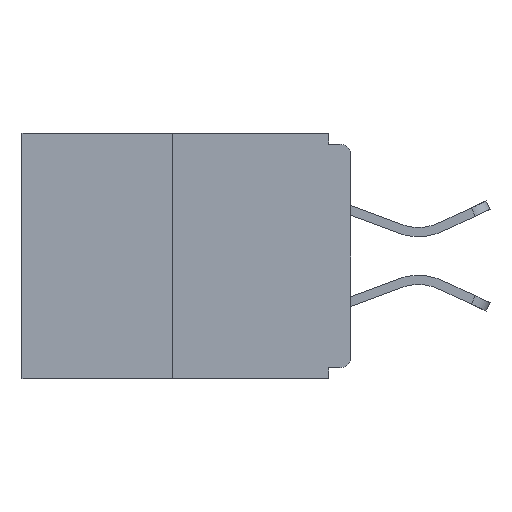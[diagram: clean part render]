
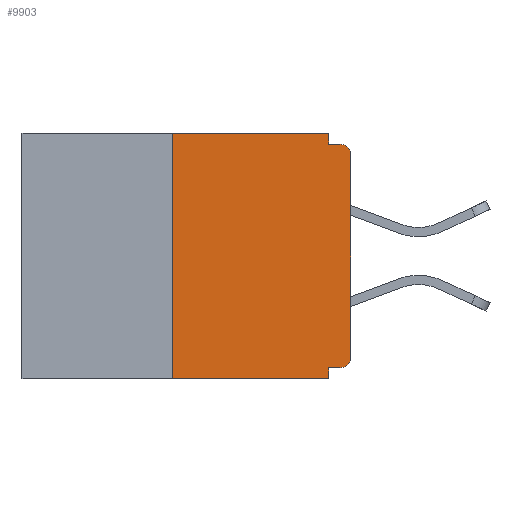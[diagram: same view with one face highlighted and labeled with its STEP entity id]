
A CAD part, left-side view. The second image highlights one B-rep face of the part: STEP entity #9903.
In plain terms, the highlighted planar face has unit normal (-1, 0, 0).
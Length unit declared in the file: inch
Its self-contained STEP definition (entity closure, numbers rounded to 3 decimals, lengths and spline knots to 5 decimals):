
#347 = LINE ( 'NONE', #2118, #11149 ) ;
#671 = EDGE_CURVE ( 'NONE', #13263, #13333, #12564, .T. ) ;
#1128 = PLANE ( 'NONE',  #15144 ) ;
#1147 = DIRECTION ( 'NONE',  ( 0., -1., 0. ) ) ;
#1541 = DIRECTION ( 'NONE',  ( -1., 0., 0. ) ) ;
#1596 = VERTEX_POINT ( 'NONE', #17377 ) ;
#2118 = CARTESIAN_POINT ( 'NONE',  ( 0., 0., -0.015 ) ) ;
#2315 = EDGE_CURVE ( 'NONE', #16190, #14720, #13131, .T. ) ;
#2697 = EDGE_CURVE ( 'NONE', #3574, #12974, #347, .T. ) ;
#3003 = CARTESIAN_POINT ( 'NONE',  ( 0., 0.015, -0.328 ) ) ;
#3574 = VERTEX_POINT ( 'NONE', #13955 ) ;
#3679 = VECTOR ( 'NONE', #7812, 39.37008 ) ;
#4064 = ORIENTED_EDGE ( 'NONE', *, *, #4828, .T. ) ;
#4545 = VECTOR ( 'NONE', #11981, 39.37008 ) ;
#4656 = FACE_OUTER_BOUND ( 'NONE', #7169, .T. ) ;
#4782 = DIRECTION ( 'NONE',  ( 0., 0., -1. ) ) ;
#4828 = EDGE_CURVE ( 'NONE', #16190, #13263, #16814, .T. ) ;
#5537 = CARTESIAN_POINT ( 'NONE',  ( 0., 0., -0.03 ) ) ;
#6177 = CARTESIAN_POINT ( 'NONE',  ( 0., 0.46, 0. ) ) ;
#6214 = DIRECTION ( 'NONE',  ( -1., 0., 0. ) ) ;
#6515 = DIRECTION ( 'NONE',  ( 0., 0., 1. ) ) ;
#6695 = DIRECTION ( 'NONE',  ( 0., 0., -1. ) ) ;
#7169 = EDGE_LOOP ( 'NONE', ( #10164, #13469, #17278, #12379, #13706, #4064, #12272, #15952, #9424, #13697 ) ) ;
#7199 = EDGE_CURVE ( 'NONE', #1596, #9937, #8522, .T. ) ;
#7812 = DIRECTION ( 'NONE',  ( 0., 0., -1. ) ) ;
#8417 = EDGE_CURVE ( 'NONE', #1596, #10927, #14379, .T. ) ;
#8522 = LINE ( 'NONE', #10633, #4545 ) ;
#8902 = EDGE_CURVE ( 'NONE', #14720, #10927, #15701, .T. ) ;
#9424 = ORIENTED_EDGE ( 'NONE', *, *, #2697, .F. ) ;
#9737 = CARTESIAN_POINT ( 'NONE',  ( 0., 0.46, -0.343 ) ) ;
#9903 = ADVANCED_FACE ( 'NONE', ( #4656 ), #1128, .F. ) ;
#9907 = LINE ( 'NONE', #6177, #15163 ) ;
#9937 = VERTEX_POINT ( 'NONE', #15411 ) ;
#9970 = CARTESIAN_POINT ( 'NONE',  ( 0., 0.031, 0. ) ) ;
#10164 = ORIENTED_EDGE ( 'NONE', *, *, #10720, .F. ) ;
#10177 = CARTESIAN_POINT ( 'NONE',  ( 0., 0.015, -0.03 ) ) ;
#10633 = CARTESIAN_POINT ( 'NONE',  ( 0., 0.25, 0. ) ) ;
#10720 = EDGE_CURVE ( 'NONE', #9937, #13345, #9907, .T. ) ;
#10927 = VERTEX_POINT ( 'NONE', #17687 ) ;
#10997 = CARTESIAN_POINT ( 'NONE',  ( 0., 0.46, 0. ) ) ;
#11007 = CARTESIAN_POINT ( 'NONE',  ( 0., 0.015, -0.015 ) ) ;
#11015 = CARTESIAN_POINT ( 'NONE',  ( 0., 0., -0.328 ) ) ;
#11149 = VECTOR ( 'NONE', #11912, 39.37008 ) ;
#11470 = EDGE_CURVE ( 'NONE', #13333, #12974, #12942, .T. ) ;
#11912 = DIRECTION ( 'NONE',  ( 0., -1., 0. ) ) ;
#11981 = DIRECTION ( 'NONE',  ( 0., 0., 1. ) ) ;
#12065 = CARTESIAN_POINT ( 'NONE',  ( 0., 0.031, -0.343 ) ) ;
#12092 = EDGE_CURVE ( 'NONE', #13345, #3574, #15109, .T. ) ;
#12272 = ORIENTED_EDGE ( 'NONE', *, *, #671, .T. ) ;
#12313 = DIRECTION ( 'NONE',  ( 0., 1., 0. ) ) ;
#12379 = ORIENTED_EDGE ( 'NONE', *, *, #8902, .F. ) ;
#12489 = CARTESIAN_POINT ( 'NONE',  ( 0., 0., -0.313 ) ) ;
#12564 = LINE ( 'NONE', #13523, #18075 ) ;
#12942 = CIRCLE ( 'NONE', #17779, 0.015 ) ;
#12974 = VERTEX_POINT ( 'NONE', #11007 ) ;
#13131 = LINE ( 'NONE', #11015, #15108 ) ;
#13263 = VERTEX_POINT ( 'NONE', #12489 ) ;
#13333 = VERTEX_POINT ( 'NONE', #5537 ) ;
#13345 = VERTEX_POINT ( 'NONE', #9970 ) ;
#13469 = ORIENTED_EDGE ( 'NONE', *, *, #7199, .F. ) ;
#13523 = CARTESIAN_POINT ( 'NONE',  ( 0., 0., 0. ) ) ;
#13697 = ORIENTED_EDGE ( 'NONE', *, *, #12092, .F. ) ;
#13706 = ORIENTED_EDGE ( 'NONE', *, *, #2315, .F. ) ;
#13955 = CARTESIAN_POINT ( 'NONE',  ( 0., 0.031, -0.015 ) ) ;
#14379 = LINE ( 'NONE', #9737, #16824 ) ;
#14720 = VERTEX_POINT ( 'NONE', #16322 ) ;
#14875 = DIRECTION ( 'NONE',  ( 0., 0., -1. ) ) ;
#15108 = VECTOR ( 'NONE', #12313, 39.37008 ) ;
#15109 = LINE ( 'NONE', #16243, #3679 ) ;
#15144 = AXIS2_PLACEMENT_3D ( 'NONE', #10997, #15344, #6695 ) ;
#15163 = VECTOR ( 'NONE', #16266, 39.37008 ) ;
#15344 = DIRECTION ( 'NONE',  ( 1., 0., 0. ) ) ;
#15411 = CARTESIAN_POINT ( 'NONE',  ( 0., 0.25, 0. ) ) ;
#15701 = LINE ( 'NONE', #12065, #16808 ) ;
#15952 = ORIENTED_EDGE ( 'NONE', *, *, #11470, .T. ) ;
#16190 = VERTEX_POINT ( 'NONE', #3003 ) ;
#16243 = CARTESIAN_POINT ( 'NONE',  ( 0., 0.031, 0. ) ) ;
#16266 = DIRECTION ( 'NONE',  ( 0., -1., 0. ) ) ;
#16322 = CARTESIAN_POINT ( 'NONE',  ( 0., 0.031, -0.328 ) ) ;
#16808 = VECTOR ( 'NONE', #14875, 39.37008 ) ;
#16814 = CIRCLE ( 'NONE', #17317, 0.015 ) ;
#16824 = VECTOR ( 'NONE', #1147, 39.37008 ) ;
#16983 = CARTESIAN_POINT ( 'NONE',  ( 0., 0.015, -0.313 ) ) ;
#17244 = DIRECTION ( 'NONE',  ( 0., 0., -1. ) ) ;
#17278 = ORIENTED_EDGE ( 'NONE', *, *, #8417, .T. ) ;
#17317 = AXIS2_PLACEMENT_3D ( 'NONE', #16983, #6214, #4782 ) ;
#17377 = CARTESIAN_POINT ( 'NONE',  ( 0., 0.25, -0.343 ) ) ;
#17687 = CARTESIAN_POINT ( 'NONE',  ( 0., 0.031, -0.343 ) ) ;
#17779 = AXIS2_PLACEMENT_3D ( 'NONE', #10177, #1541, #17244 ) ;
#18075 = VECTOR ( 'NONE', #6515, 39.37008 ) ;
